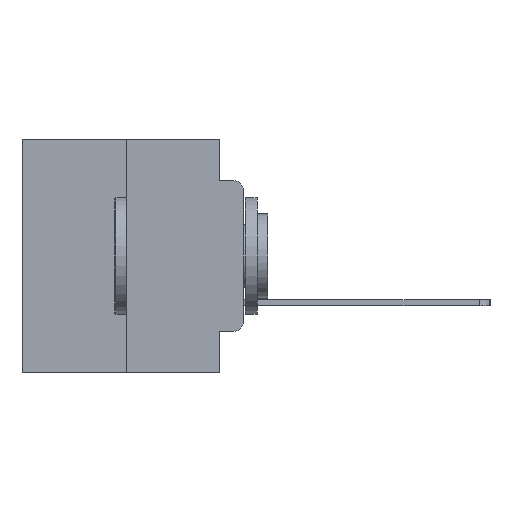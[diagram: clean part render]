
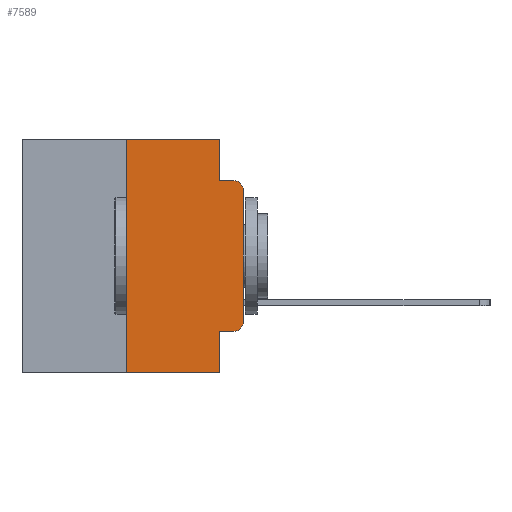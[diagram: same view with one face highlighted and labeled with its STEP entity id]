
A CAD part, left-side view. The second image highlights one B-rep face of the part: STEP entity #7589.
In plain terms, the highlighted planar face has unit normal (-1, 0, 0).
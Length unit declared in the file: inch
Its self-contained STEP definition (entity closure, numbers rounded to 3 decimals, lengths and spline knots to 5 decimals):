
#295 = EDGE_CURVE ( 'NONE', #21711, #17673, #13523, .T. ) ;
#638 = ORIENTED_EDGE ( 'NONE', *, *, #12632, .F. ) ;
#1278 = ORIENTED_EDGE ( 'NONE', *, *, #5759, .F. ) ;
#1358 = ORIENTED_EDGE ( 'NONE', *, *, #295, .F. ) ;
#1601 = CARTESIAN_POINT ( 'NONE',  ( 0., 0.051, -0.0885 ) ) ;
#2271 = ORIENTED_EDGE ( 'NONE', *, *, #4739, .T. ) ;
#2612 = CARTESIAN_POINT ( 'NONE',  ( 0., 0.02, -0.4115 ) ) ;
#2706 = ORIENTED_EDGE ( 'NONE', *, *, #20066, .F. ) ;
#2997 = DIRECTION ( 'NONE',  ( 0., 0., -1. ) ) ;
#3126 = VECTOR ( 'NONE', #8269, 39.37008 ) ;
#3254 = ORIENTED_EDGE ( 'NONE', *, *, #17656, .T. ) ;
#3306 = CIRCLE ( 'NONE', #10136, 0.02 ) ;
#3343 = ORIENTED_EDGE ( 'NONE', *, *, #23526, .T. ) ;
#3427 = CARTESIAN_POINT ( 'NONE',  ( 0., 0.02, -0.1085 ) ) ;
#3916 = VECTOR ( 'NONE', #5953, 39.37008 ) ;
#4739 = EDGE_CURVE ( 'NONE', #21711, #17277, #13683, .T. ) ;
#5235 = VERTEX_POINT ( 'NONE', #1601 ) ;
#5671 = DIRECTION ( 'NONE',  ( 0., 0., -1. ) ) ;
#5754 = LINE ( 'NONE', #8366, #11251 ) ;
#5759 = EDGE_CURVE ( 'NONE', #17673, #9980, #8859, .T. ) ;
#5953 = DIRECTION ( 'NONE',  ( 0., -1., 0. ) ) ;
#7169 = DIRECTION ( 'NONE',  ( 0., -1., 0. ) ) ;
#7261 = CARTESIAN_POINT ( 'NONE',  ( 0., 0.25, 0. ) ) ;
#7362 = LINE ( 'NONE', #18349, #8026 ) ;
#7468 = VECTOR ( 'NONE', #22776, 39.37008 ) ;
#7589 = ADVANCED_FACE ( 'NONE', ( #13213 ), #13464, .F. ) ;
#7825 = VECTOR ( 'NONE', #10451, 39.37008 ) ;
#7882 = EDGE_CURVE ( 'NONE', #14477, #15718, #7362, .T. ) ;
#8026 = VECTOR ( 'NONE', #8364, 39.37008 ) ;
#8269 = DIRECTION ( 'NONE',  ( 0., -1., 0. ) ) ;
#8364 = DIRECTION ( 'NONE',  ( 0., 0., 1. ) ) ;
#8366 = CARTESIAN_POINT ( 'NONE',  ( 0., 0.051, 0. ) ) ;
#8859 = LINE ( 'NONE', #22292, #3126 ) ;
#9019 = VERTEX_POINT ( 'NONE', #2612 ) ;
#9199 = DIRECTION ( 'NONE',  ( -1., 0., 0. ) ) ;
#9823 = AXIS2_PLACEMENT_3D ( 'NONE', #23317, #15444, #2997 ) ;
#9980 = VERTEX_POINT ( 'NONE', #25906 ) ;
#10136 = AXIS2_PLACEMENT_3D ( 'NONE', #3427, #17770, #5671 ) ;
#10451 = DIRECTION ( 'NONE',  ( 0., 0., -1. ) ) ;
#11145 = VECTOR ( 'NONE', #15625, 39.37008 ) ;
#11251 = VECTOR ( 'NONE', #22388, 39.37008 ) ;
#11296 = CARTESIAN_POINT ( 'NONE',  ( 0., 0., -0.3915 ) ) ;
#11595 = CARTESIAN_POINT ( 'NONE',  ( 0., 0.051, -0.0885 ) ) ;
#11809 = CARTESIAN_POINT ( 'NONE',  ( 0., 0., -0.1085 ) ) ;
#12342 = EDGE_LOOP ( 'NONE', ( #25762, #17134, #22459, #638, #1278, #1358, #2271, #2706, #3254, #3343 ) ) ;
#12427 = LINE ( 'NONE', #11595, #11145 ) ;
#12632 = EDGE_CURVE ( 'NONE', #9980, #5235, #13852, .T. ) ;
#13213 = FACE_OUTER_BOUND ( 'NONE', #12342, .T. ) ;
#13342 = VECTOR ( 'NONE', #7169, 39.37008 ) ;
#13464 = PLANE ( 'NONE',  #9823 ) ;
#13523 = LINE ( 'NONE', #17340, #7468 ) ;
#13683 = LINE ( 'NONE', #23966, #3916 ) ;
#13852 = LINE ( 'NONE', #22407, #7825 ) ;
#14275 = CARTESIAN_POINT ( 'NONE',  ( 0., 0.051, -0.5 ) ) ;
#14477 = VERTEX_POINT ( 'NONE', #11296 ) ;
#15444 = DIRECTION ( 'NONE',  ( 1., 0., 0. ) ) ;
#15625 = DIRECTION ( 'NONE',  ( 0., -1., 0. ) ) ;
#15718 = VERTEX_POINT ( 'NONE', #11809 ) ;
#16698 = VERTEX_POINT ( 'NONE', #18343 ) ;
#17134 = ORIENTED_EDGE ( 'NONE', *, *, #21095, .T. ) ;
#17277 = VERTEX_POINT ( 'NONE', #14275 ) ;
#17340 = CARTESIAN_POINT ( 'NONE',  ( 0., 0.25, 0. ) ) ;
#17656 = EDGE_CURVE ( 'NONE', #16698, #9019, #24461, .T. ) ;
#17673 = VERTEX_POINT ( 'NONE', #7261 ) ;
#17770 = DIRECTION ( 'NONE',  ( -1., 0., 0. ) ) ;
#17996 = CARTESIAN_POINT ( 'NONE',  ( 0., 0.25, -0.5 ) ) ;
#18036 = CARTESIAN_POINT ( 'NONE',  ( 0., 0.02, -0.0885 ) ) ;
#18343 = CARTESIAN_POINT ( 'NONE',  ( 0., 0.051, -0.4115 ) ) ;
#18349 = CARTESIAN_POINT ( 'NONE',  ( 0., 0., 0. ) ) ;
#18670 = AXIS2_PLACEMENT_3D ( 'NONE', #21164, #9199, #23129 ) ;
#19150 = CIRCLE ( 'NONE', #18670, 0.02 ) ;
#20066 = EDGE_CURVE ( 'NONE', #16698, #17277, #5754, .T. ) ;
#21095 = EDGE_CURVE ( 'NONE', #15718, #22340, #3306, .T. ) ;
#21164 = CARTESIAN_POINT ( 'NONE',  ( 0., 0.02, -0.3915 ) ) ;
#21711 = VERTEX_POINT ( 'NONE', #17996 ) ;
#22292 = CARTESIAN_POINT ( 'NONE',  ( 0., 0.473, 0. ) ) ;
#22340 = VERTEX_POINT ( 'NONE', #18036 ) ;
#22388 = DIRECTION ( 'NONE',  ( 0., 0., -1. ) ) ;
#22407 = CARTESIAN_POINT ( 'NONE',  ( 0., 0.051, 0. ) ) ;
#22459 = ORIENTED_EDGE ( 'NONE', *, *, #25821, .F. ) ;
#22776 = DIRECTION ( 'NONE',  ( 0., 0., 1. ) ) ;
#23102 = CARTESIAN_POINT ( 'NONE',  ( 0., 0.051, -0.4115 ) ) ;
#23129 = DIRECTION ( 'NONE',  ( 0., 0., -1. ) ) ;
#23317 = CARTESIAN_POINT ( 'NONE',  ( 0., 0.473, 0. ) ) ;
#23526 = EDGE_CURVE ( 'NONE', #9019, #14477, #19150, .T. ) ;
#23966 = CARTESIAN_POINT ( 'NONE',  ( 0., 0.473, -0.5 ) ) ;
#24461 = LINE ( 'NONE', #23102, #13342 ) ;
#25762 = ORIENTED_EDGE ( 'NONE', *, *, #7882, .T. ) ;
#25821 = EDGE_CURVE ( 'NONE', #5235, #22340, #12427, .T. ) ;
#25906 = CARTESIAN_POINT ( 'NONE',  ( 0., 0.051, 0. ) ) ;
